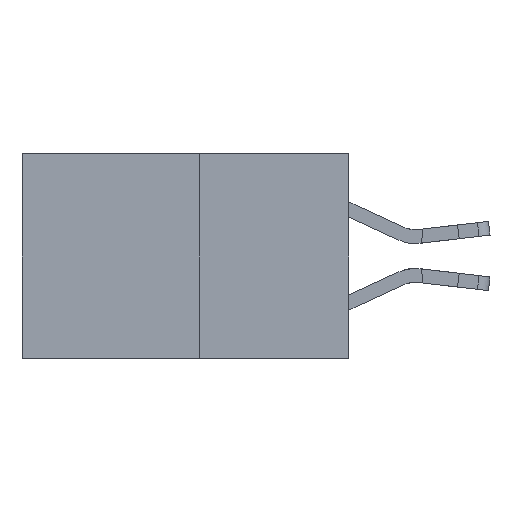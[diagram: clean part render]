
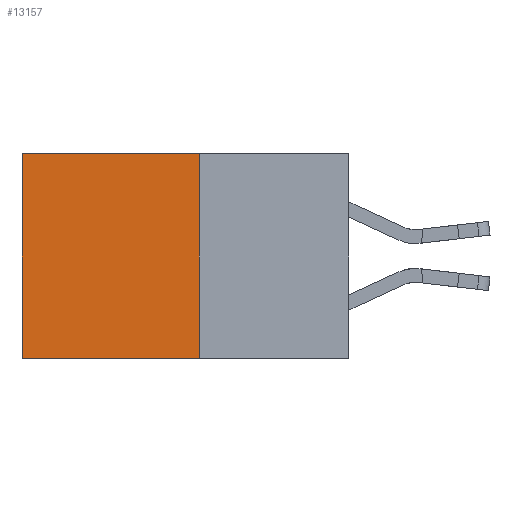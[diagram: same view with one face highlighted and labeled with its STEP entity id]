
A CAD part, left-side view. The second image highlights one B-rep face of the part: STEP entity #13157.
In plain terms, the highlighted planar face has unit normal (-1, 0, 0).
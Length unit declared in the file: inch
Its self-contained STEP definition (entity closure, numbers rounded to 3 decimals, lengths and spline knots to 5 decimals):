
#3999 = PLANE ( 'NONE',  #6966 ) ;
#4640 = VERTEX_POINT ( 'NONE', #28133 ) ;
#4751 = LINE ( 'NONE', #24076, #23802 ) ;
#4821 = EDGE_CURVE ( 'NONE', #4640, #16826, #4916, .T. ) ;
#4916 = LINE ( 'NONE', #22231, #22480 ) ;
#4993 = DIRECTION ( 'NONE',  ( 0., 0., -1. ) ) ;
#6319 = VERTEX_POINT ( 'NONE', #16374 ) ;
#6397 = LINE ( 'NONE', #18862, #30146 ) ;
#6432 = CARTESIAN_POINT ( 'NONE',  ( 0.277, 0.27, -0.37 ) ) ;
#6966 = AXIS2_PLACEMENT_3D ( 'NONE', #6432, #8772, #25500 ) ;
#6969 = EDGE_CURVE ( 'NONE', #4640, #9061, #7001, .T. ) ;
#7001 = LINE ( 'NONE', #13907, #25293 ) ;
#8772 = DIRECTION ( 'NONE',  ( 1., 0., 0. ) ) ;
#9061 = VERTEX_POINT ( 'NONE', #19136 ) ;
#11809 = ORIENTED_EDGE ( 'NONE', *, *, #4821, .T. ) ;
#12868 = ORIENTED_EDGE ( 'NONE', *, *, #17258, .T. ) ;
#13157 = ADVANCED_FACE ( 'NONE', ( #17266 ), #3999, .F. ) ;
#13330 = EDGE_CURVE ( 'NONE', #9061, #6319, #6397, .T. ) ;
#13907 = CARTESIAN_POINT ( 'NONE',  ( 0.277, 0.27, -0.37 ) ) ;
#15469 = ORIENTED_EDGE ( 'NONE', *, *, #13330, .F. ) ;
#15623 = CARTESIAN_POINT ( 'NONE',  ( 0.277, 0.59, 0. ) ) ;
#16374 = CARTESIAN_POINT ( 'NONE',  ( 0.277, 0.59, -0.37 ) ) ;
#16826 = VERTEX_POINT ( 'NONE', #15623 ) ;
#17258 = EDGE_CURVE ( 'NONE', #16826, #6319, #4751, .T. ) ;
#17266 = FACE_OUTER_BOUND ( 'NONE', #26542, .T. ) ;
#18862 = CARTESIAN_POINT ( 'NONE',  ( 0.277, 0.27, -0.37 ) ) ;
#19136 = CARTESIAN_POINT ( 'NONE',  ( 0.277, 0.27, -0.37 ) ) ;
#19527 = DIRECTION ( 'NONE',  ( 0., 0., -1. ) ) ;
#21256 = DIRECTION ( 'NONE',  ( 0., 1., 0. ) ) ;
#21856 = ORIENTED_EDGE ( 'NONE', *, *, #6969, .F. ) ;
#22231 = CARTESIAN_POINT ( 'NONE',  ( 0.277, 0.27, 0. ) ) ;
#22480 = VECTOR ( 'NONE', #28269, 39.37008 ) ;
#23802 = VECTOR ( 'NONE', #4993, 39.37008 ) ;
#24076 = CARTESIAN_POINT ( 'NONE',  ( 0.277, 0.59, -0.37 ) ) ;
#25293 = VECTOR ( 'NONE', #19527, 39.37008 ) ;
#25500 = DIRECTION ( 'NONE',  ( 0., 0., -1. ) ) ;
#26542 = EDGE_LOOP ( 'NONE', ( #12868, #15469, #21856, #11809 ) ) ;
#28133 = CARTESIAN_POINT ( 'NONE',  ( 0.277, 0.27, 0. ) ) ;
#28269 = DIRECTION ( 'NONE',  ( 0., 1., 0. ) ) ;
#30146 = VECTOR ( 'NONE', #21256, 39.37008 ) ;
